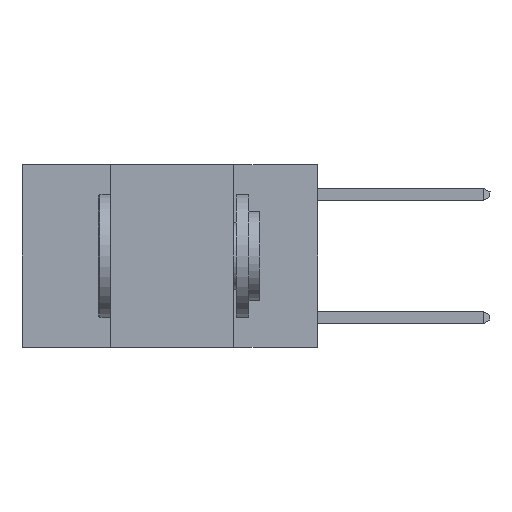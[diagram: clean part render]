
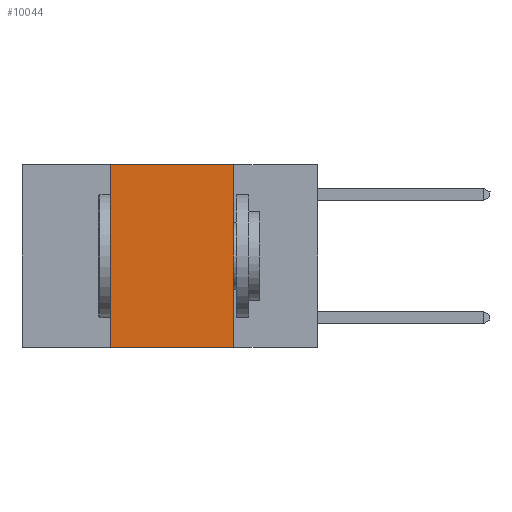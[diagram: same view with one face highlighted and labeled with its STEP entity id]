
A CAD part, left-side view. The second image highlights one B-rep face of the part: STEP entity #10044.
In plain terms, the highlighted planar face has unit normal (-1, 0, 0).
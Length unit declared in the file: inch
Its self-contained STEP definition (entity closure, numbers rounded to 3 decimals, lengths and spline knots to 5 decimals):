
#233 = LINE ( 'NONE', #9902, #20727 ) ;
#757 = CARTESIAN_POINT ( 'NONE',  ( 0., 0.6, 0. ) ) ;
#861 = VERTEX_POINT ( 'NONE', #9362 ) ;
#1263 = ORIENTED_EDGE ( 'NONE', *, *, #16993, .F. ) ;
#1283 = DIRECTION ( 'NONE',  ( 0., 0., 1. ) ) ;
#2519 = VERTEX_POINT ( 'NONE', #23474 ) ;
#2542 = DIRECTION ( 'NONE',  ( 1., 0., 0. ) ) ;
#3413 = DIRECTION ( 'NONE',  ( 0., -1., 0. ) ) ;
#3867 = CARTESIAN_POINT ( 'NONE',  ( 0., 0.17, -0.37 ) ) ;
#5385 = AXIS2_PLACEMENT_3D ( 'NONE', #757, #2542, #15953 ) ;
#6591 = VERTEX_POINT ( 'NONE', #3867 ) ;
#7449 = EDGE_CURVE ( 'NONE', #2519, #6591, #21122, .T. ) ;
#8184 = CARTESIAN_POINT ( 'NONE',  ( 0., 0.6, 0. ) ) ;
#9256 = CARTESIAN_POINT ( 'NONE',  ( 0., 0.42, 0. ) ) ;
#9362 = CARTESIAN_POINT ( 'NONE',  ( 0., 0.17, 0. ) ) ;
#9902 = CARTESIAN_POINT ( 'NONE',  ( 0., 0.17, 0. ) ) ;
#10044 = ADVANCED_FACE ( 'NONE', ( #20385 ), #18449, .F. ) ;
#10595 = VECTOR ( 'NONE', #1283, 39.37008 ) ;
#11509 = VERTEX_POINT ( 'NONE', #20369 ) ;
#11558 = EDGE_LOOP ( 'NONE', ( #19388, #12440, #1263, #13028 ) ) ;
#11570 = EDGE_CURVE ( 'NONE', #861, #6591, #233, .T. ) ;
#12077 = LINE ( 'NONE', #8184, #17009 ) ;
#12440 = ORIENTED_EDGE ( 'NONE', *, *, #17642, .F. ) ;
#13028 = ORIENTED_EDGE ( 'NONE', *, *, #7449, .T. ) ;
#13883 = DIRECTION ( 'NONE',  ( 0., -1., 0. ) ) ;
#15953 = DIRECTION ( 'NONE',  ( 0., 0., -1. ) ) ;
#16993 = EDGE_CURVE ( 'NONE', #2519, #11509, #18960, .T. ) ;
#17009 = VECTOR ( 'NONE', #13883, 39.37008 ) ;
#17642 = EDGE_CURVE ( 'NONE', #11509, #861, #12077, .T. ) ;
#18449 = PLANE ( 'NONE',  #5385 ) ;
#18960 = LINE ( 'NONE', #9256, #10595 ) ;
#19147 = CARTESIAN_POINT ( 'NONE',  ( 0., 0.6, -0.37 ) ) ;
#19388 = ORIENTED_EDGE ( 'NONE', *, *, #11570, .F. ) ;
#20369 = CARTESIAN_POINT ( 'NONE',  ( 0., 0.42, 0. ) ) ;
#20385 = FACE_OUTER_BOUND ( 'NONE', #11558, .T. ) ;
#20727 = VECTOR ( 'NONE', #24289, 39.37008 ) ;
#21122 = LINE ( 'NONE', #19147, #23129 ) ;
#23129 = VECTOR ( 'NONE', #3413, 39.37008 ) ;
#23474 = CARTESIAN_POINT ( 'NONE',  ( 0., 0.42, -0.37 ) ) ;
#24289 = DIRECTION ( 'NONE',  ( 0., 0., -1. ) ) ;
